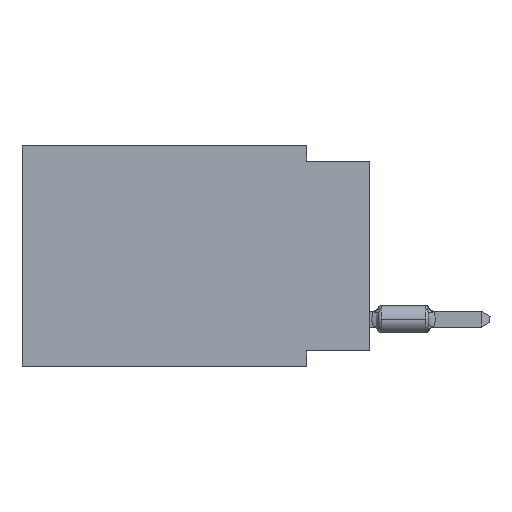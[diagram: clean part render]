
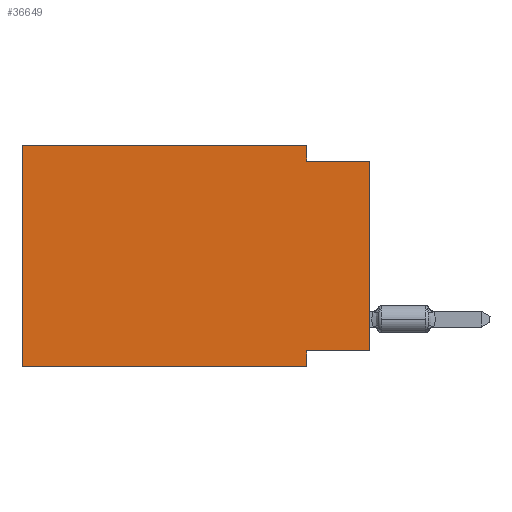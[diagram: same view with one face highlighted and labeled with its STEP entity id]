
A CAD part, left-side view. The second image highlights one B-rep face of the part: STEP entity #36649.
In plain terms, the highlighted planar face has unit normal (-1, 0, 0).
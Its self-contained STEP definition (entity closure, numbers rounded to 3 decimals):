
#343 = VERTEX_POINT ( 'NONE', #24247 ) ;
#724 = AXIS2_PLACEMENT_3D ( 'NONE', #18549, #34321, #30422 ) ;
#1536 = EDGE_CURVE ( 'NONE', #7503, #47284, #39785, .T. ) ;
#2770 = PLANE ( 'NONE',  #724 ) ;
#4421 = DIRECTION ( 'NONE',  ( 0., -1., 0. ) ) ;
#5310 = EDGE_CURVE ( 'NONE', #47284, #20910, #30021, .T. ) ;
#5409 = LINE ( 'NONE', #16056, #13251 ) ;
#5982 = EDGE_CURVE ( 'NONE', #343, #46918, #38290, .T. ) ;
#6203 = CARTESIAN_POINT ( 'NONE',  ( 0., 2.54, 0. ) ) ;
#6352 = DIRECTION ( 'NONE',  ( 0., 0., -1. ) ) ;
#6995 = CARTESIAN_POINT ( 'NONE',  ( 0., 2.54, 0. ) ) ;
#7503 = VERTEX_POINT ( 'NONE', #36265 ) ;
#8780 = CARTESIAN_POINT ( 'NONE',  ( 0., 2.54, -8.255 ) ) ;
#9585 = CARTESIAN_POINT ( 'NONE',  ( 0., 0., -0.635 ) ) ;
#10691 = VECTOR ( 'NONE', #17886, 1000. ) ;
#10800 = VECTOR ( 'NONE', #19145, 1000. ) ;
#10878 = ORIENTED_EDGE ( 'NONE', *, *, #1536, .F. ) ;
#11084 = EDGE_CURVE ( 'NONE', #33515, #47594, #13868, .T. ) ;
#11506 = DIRECTION ( 'NONE',  ( 0., 1., 0. ) ) ;
#13251 = VECTOR ( 'NONE', #47851, 1000. ) ;
#13660 = CARTESIAN_POINT ( 'NONE',  ( 0., 2.54, -8.89 ) ) ;
#13702 = VECTOR ( 'NONE', #11506, 1000. ) ;
#13868 = LINE ( 'NONE', #37652, #24985 ) ;
#15215 = EDGE_CURVE ( 'NONE', #20910, #46918, #32602, .T. ) ;
#16056 = CARTESIAN_POINT ( 'NONE',  ( 0., 13.97, 0. ) ) ;
#17654 = DIRECTION ( 'NONE',  ( 0., -1., 0. ) ) ;
#17886 = DIRECTION ( 'NONE',  ( 0., 0., -1. ) ) ;
#18424 = CARTESIAN_POINT ( 'NONE',  ( 0., 0., -0.635 ) ) ;
#18549 = CARTESIAN_POINT ( 'NONE',  ( 0., 13.97, 0. ) ) ;
#19145 = DIRECTION ( 'NONE',  ( 0., 0., 1. ) ) ;
#19829 = VECTOR ( 'NONE', #17654, 1000. ) ;
#20910 = VERTEX_POINT ( 'NONE', #36656 ) ;
#24247 = CARTESIAN_POINT ( 'NONE',  ( 0., 0., -8.255 ) ) ;
#24592 = CARTESIAN_POINT ( 'NONE',  ( 0., 0., -8.255 ) ) ;
#24985 = VECTOR ( 'NONE', #6352, 1000. ) ;
#25708 = ORIENTED_EDGE ( 'NONE', *, *, #45486, .T. ) ;
#25937 = ORIENTED_EDGE ( 'NONE', *, *, #15215, .F. ) ;
#28509 = LINE ( 'NONE', #36537, #19829 ) ;
#29349 = EDGE_CURVE ( 'NONE', #343, #33515, #48139, .T. ) ;
#30021 = LINE ( 'NONE', #6995, #10691 ) ;
#30422 = DIRECTION ( 'NONE',  ( 0., 0., -1. ) ) ;
#32602 = LINE ( 'NONE', #9585, #43789 ) ;
#33034 = ORIENTED_EDGE ( 'NONE', *, *, #33574, .F. ) ;
#33515 = VERTEX_POINT ( 'NONE', #8780 ) ;
#33574 = EDGE_CURVE ( 'NONE', #42694, #7503, #5409, .T. ) ;
#33946 = EDGE_LOOP ( 'NONE', ( #34199, #25937, #39088, #10878, #33034, #25708, #36844, #49784 ) ) ;
#34199 = ORIENTED_EDGE ( 'NONE', *, *, #5982, .T. ) ;
#34321 = DIRECTION ( 'NONE',  ( 1., 0., 0. ) ) ;
#36059 = VECTOR ( 'NONE', #44176, 1000. ) ;
#36265 = CARTESIAN_POINT ( 'NONE',  ( 0., 13.97, 0. ) ) ;
#36537 = CARTESIAN_POINT ( 'NONE',  ( 0., 13.97, -8.89 ) ) ;
#36649 = ADVANCED_FACE ( 'NONE', ( #38196 ), #2770, .F. ) ;
#36656 = CARTESIAN_POINT ( 'NONE',  ( 0., 2.54, -0.635 ) ) ;
#36668 = CARTESIAN_POINT ( 'NONE',  ( 0., 13.97, 0. ) ) ;
#36844 = ORIENTED_EDGE ( 'NONE', *, *, #11084, .F. ) ;
#37652 = CARTESIAN_POINT ( 'NONE',  ( 0., 2.54, -8.89 ) ) ;
#38196 = FACE_OUTER_BOUND ( 'NONE', #33946, .T. ) ;
#38290 = LINE ( 'NONE', #42169, #10800 ) ;
#39040 = CARTESIAN_POINT ( 'NONE',  ( 0., 13.97, -8.89 ) ) ;
#39088 = ORIENTED_EDGE ( 'NONE', *, *, #5310, .F. ) ;
#39785 = LINE ( 'NONE', #36668, #36059 ) ;
#42169 = CARTESIAN_POINT ( 'NONE',  ( 0., 0., 0. ) ) ;
#42694 = VERTEX_POINT ( 'NONE', #39040 ) ;
#43789 = VECTOR ( 'NONE', #4421, 1000. ) ;
#44176 = DIRECTION ( 'NONE',  ( 0., -1., 0. ) ) ;
#45486 = EDGE_CURVE ( 'NONE', #42694, #47594, #28509, .T. ) ;
#46918 = VERTEX_POINT ( 'NONE', #18424 ) ;
#47284 = VERTEX_POINT ( 'NONE', #6203 ) ;
#47594 = VERTEX_POINT ( 'NONE', #13660 ) ;
#47851 = DIRECTION ( 'NONE',  ( 0., 0., 1. ) ) ;
#48139 = LINE ( 'NONE', #24592, #13702 ) ;
#49784 = ORIENTED_EDGE ( 'NONE', *, *, #29349, .F. ) ;
